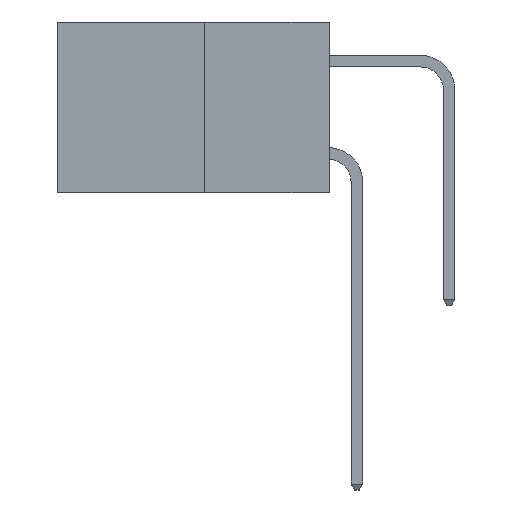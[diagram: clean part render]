
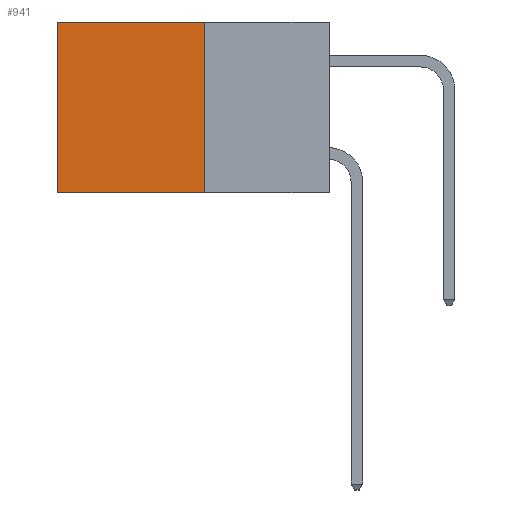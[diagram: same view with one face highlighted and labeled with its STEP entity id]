
A CAD part, left-side view. The second image highlights one B-rep face of the part: STEP entity #941.
In plain terms, the highlighted planar face has unit normal (-1, 0, 0).
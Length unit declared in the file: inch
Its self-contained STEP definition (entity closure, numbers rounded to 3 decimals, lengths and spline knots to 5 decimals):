
#38 = LINE ( 'NONE', #6600, #11173 ) ;
#65 = CARTESIAN_POINT ( 'NONE',  ( 0.277, 0.27, 0. ) ) ;
#458 = ORIENTED_EDGE ( 'NONE', *, *, #10048, .T. ) ;
#499 = DIRECTION ( 'NONE',  ( 0., 1., 0. ) ) ;
#510 = ORIENTED_EDGE ( 'NONE', *, *, #7723, .F. ) ;
#580 = CARTESIAN_POINT ( 'NONE',  ( 0.277, 0.59, -0.37 ) ) ;
#618 = ORIENTED_EDGE ( 'NONE', *, *, #2477, .F. ) ;
#860 = CARTESIAN_POINT ( 'NONE',  ( 0.277, 0.27, -0.37 ) ) ;
#891 = EDGE_CURVE ( 'NONE', #7926, #5156, #2847, .T. ) ;
#941 = ADVANCED_FACE ( 'NONE', ( #4716 ), #6580, .F. ) ;
#1016 = ORIENTED_EDGE ( 'NONE', *, *, #891, .T. ) ;
#1075 = DIRECTION ( 'NONE',  ( 0., 1., 0. ) ) ;
#1748 = CARTESIAN_POINT ( 'NONE',  ( 0.277, 0.27, -0.37 ) ) ;
#2110 = DIRECTION ( 'NONE',  ( 0., 0., -1. ) ) ;
#2477 = EDGE_CURVE ( 'NONE', #7926, #8553, #10987, .T. ) ;
#2669 = DIRECTION ( 'NONE',  ( 0., 0., -1. ) ) ;
#2838 = DIRECTION ( 'NONE',  ( 1., 0., 0. ) ) ;
#2847 = LINE ( 'NONE', #65, #9531 ) ;
#3899 = CARTESIAN_POINT ( 'NONE',  ( 0.277, 0.27, -0.37 ) ) ;
#4716 = FACE_OUTER_BOUND ( 'NONE', #5850, .T. ) ;
#5156 = VERTEX_POINT ( 'NONE', #8463 ) ;
#5486 = LINE ( 'NONE', #6834, #7562 ) ;
#5518 = AXIS2_PLACEMENT_3D ( 'NONE', #860, #2838, #2669 ) ;
#5850 = EDGE_LOOP ( 'NONE', ( #458, #510, #618, #1016 ) ) ;
#6580 = PLANE ( 'NONE',  #5518 ) ;
#6600 = CARTESIAN_POINT ( 'NONE',  ( 0.277, 0.59, -0.37 ) ) ;
#6834 = CARTESIAN_POINT ( 'NONE',  ( 0.277, 0.27, -0.37 ) ) ;
#6873 = VECTOR ( 'NONE', #7369, 39.37008 ) ;
#6933 = VERTEX_POINT ( 'NONE', #580 ) ;
#7369 = DIRECTION ( 'NONE',  ( 0., 0., -1. ) ) ;
#7562 = VECTOR ( 'NONE', #499, 39.37008 ) ;
#7723 = EDGE_CURVE ( 'NONE', #8553, #6933, #5486, .T. ) ;
#7926 = VERTEX_POINT ( 'NONE', #7980 ) ;
#7980 = CARTESIAN_POINT ( 'NONE',  ( 0.277, 0.27, 0. ) ) ;
#8463 = CARTESIAN_POINT ( 'NONE',  ( 0.277, 0.59, 0. ) ) ;
#8553 = VERTEX_POINT ( 'NONE', #1748 ) ;
#9531 = VECTOR ( 'NONE', #1075, 39.37008 ) ;
#10048 = EDGE_CURVE ( 'NONE', #5156, #6933, #38, .T. ) ;
#10987 = LINE ( 'NONE', #3899, #6873 ) ;
#11173 = VECTOR ( 'NONE', #2110, 39.37008 ) ;
